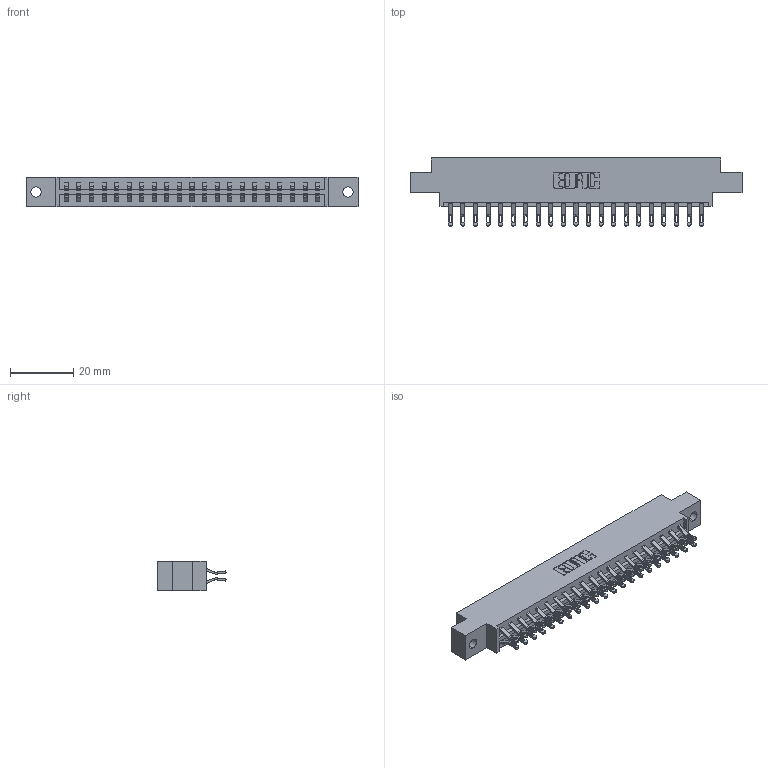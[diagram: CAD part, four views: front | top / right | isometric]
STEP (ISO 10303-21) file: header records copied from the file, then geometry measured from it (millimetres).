
FILE_DESCRIPTION (( 'STEP AP203' ), '1' );
FILE_NAME ('833-042-555-802.STEP', '2020-06-03T22:14:20', ( '' ), ( '' ), 'SwSTEP 2.0', 'SolidWorks 2020', '' );
FILE_SCHEMA (( 'CONFIG_CONTROL_DESIGN' ));
Length unit declared in the file: inch
Products named in the file (3): 345-292-001_555 Tail; 833-042-555-802; 833 Part_Offset - .128 Dia
Assembly tree (43 placements, depth 2):
  833-042-555-802
    833 Part_Offset - .128 Dia
    345-292-001_555 Tail  x42
Bounding box: 104.75 x 21.47 x 9.4 mm (x, y, z)
Volume: 10355.3 mm3; surface area: 12420 mm2
Topology: 43 solids, 43 shells, 2554 faces, 8009 edges, 5338 vertices
Faces by surface type: plane 1502, cylinder 1052
Entity records: 16687 total; most frequent: CARTESIAN_POINT 2828, ORIENTED_EDGE 2734, DIRECTION 2423, EDGE_CURVE 1367, VECTOR 1219, LINE 1219, VERTEX_POINT 910, AXIS2_PLACEMENT_3D 602
